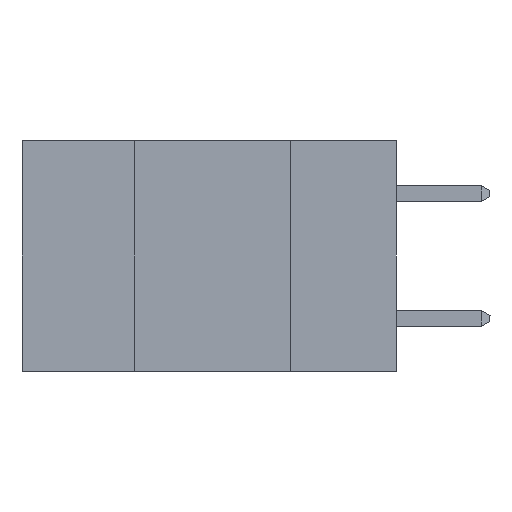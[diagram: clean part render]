
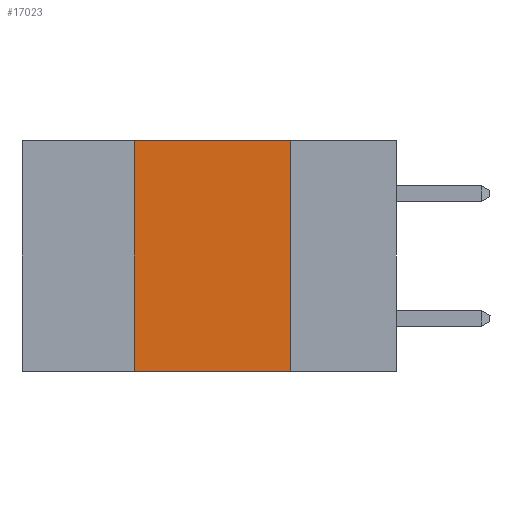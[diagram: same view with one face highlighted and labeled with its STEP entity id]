
A CAD part, left-side view. The second image highlights one B-rep face of the part: STEP entity #17023.
In plain terms, the highlighted planar face has unit normal (-1, 0, 0).
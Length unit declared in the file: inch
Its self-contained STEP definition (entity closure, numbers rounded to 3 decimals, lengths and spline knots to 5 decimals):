
#421 = EDGE_CURVE ( 'NONE', #9976, #19062, #7495, .T. ) ;
#2155 = VECTOR ( 'NONE', #16501, 39.37008 ) ;
#2731 = CARTESIAN_POINT ( 'NONE',  ( 0., 0.17, 0. ) ) ;
#3373 = CARTESIAN_POINT ( 'NONE',  ( 0., 0.42, 0. ) ) ;
#4342 = EDGE_LOOP ( 'NONE', ( #18618, #13003, #8280, #16147 ) ) ;
#4676 = DIRECTION ( 'NONE',  ( 0., 0., 1. ) ) ;
#5283 = LINE ( 'NONE', #17408, #15316 ) ;
#5982 = EDGE_CURVE ( 'NONE', #17950, #20011, #11923, .T. ) ;
#7495 = LINE ( 'NONE', #9978, #2155 ) ;
#8280 = ORIENTED_EDGE ( 'NONE', *, *, #5982, .F. ) ;
#9976 = VERTEX_POINT ( 'NONE', #2731 ) ;
#9978 = CARTESIAN_POINT ( 'NONE',  ( 0., 0.17, -0.37 ) ) ;
#10958 = DIRECTION ( 'NONE',  ( 1., 0., 0. ) ) ;
#11895 = CARTESIAN_POINT ( 'NONE',  ( 0., 0.42, -0.37 ) ) ;
#11923 = LINE ( 'NONE', #20591, #16599 ) ;
#12731 = EDGE_CURVE ( 'NONE', #20011, #9976, #5283, .T. ) ;
#13003 = ORIENTED_EDGE ( 'NONE', *, *, #12731, .F. ) ;
#13722 = CARTESIAN_POINT ( 'NONE',  ( 0., 0.6, -0.37 ) ) ;
#15230 = VECTOR ( 'NONE', #15728, 39.37008 ) ;
#15316 = VECTOR ( 'NONE', #17492, 39.37008 ) ;
#15728 = DIRECTION ( 'NONE',  ( 0., -1., 0. ) ) ;
#16147 = ORIENTED_EDGE ( 'NONE', *, *, #20131, .T. ) ;
#16501 = DIRECTION ( 'NONE',  ( 0., 0., -1. ) ) ;
#16599 = VECTOR ( 'NONE', #4676, 39.37008 ) ;
#16910 = PLANE ( 'NONE',  #22808 ) ;
#17023 = ADVANCED_FACE ( 'NONE', ( #20833 ), #16910, .F. ) ;
#17408 = CARTESIAN_POINT ( 'NONE',  ( 0., 0.6, 0. ) ) ;
#17492 = DIRECTION ( 'NONE',  ( 0., -1., 0. ) ) ;
#17950 = VERTEX_POINT ( 'NONE', #11895 ) ;
#18618 = ORIENTED_EDGE ( 'NONE', *, *, #421, .F. ) ;
#18748 = CARTESIAN_POINT ( 'NONE',  ( 0., 0.17, -0.37 ) ) ;
#19062 = VERTEX_POINT ( 'NONE', #18748 ) ;
#20011 = VERTEX_POINT ( 'NONE', #3373 ) ;
#20131 = EDGE_CURVE ( 'NONE', #17950, #19062, #25794, .T. ) ;
#20591 = CARTESIAN_POINT ( 'NONE',  ( 0., 0.42, -0.37 ) ) ;
#20833 = FACE_OUTER_BOUND ( 'NONE', #4342, .T. ) ;
#22808 = AXIS2_PLACEMENT_3D ( 'NONE', #22887, #10958, #24853 ) ;
#22887 = CARTESIAN_POINT ( 'NONE',  ( 0., 0.6, 0. ) ) ;
#24853 = DIRECTION ( 'NONE',  ( 0., 0., -1. ) ) ;
#25794 = LINE ( 'NONE', #13722, #15230 ) ;
